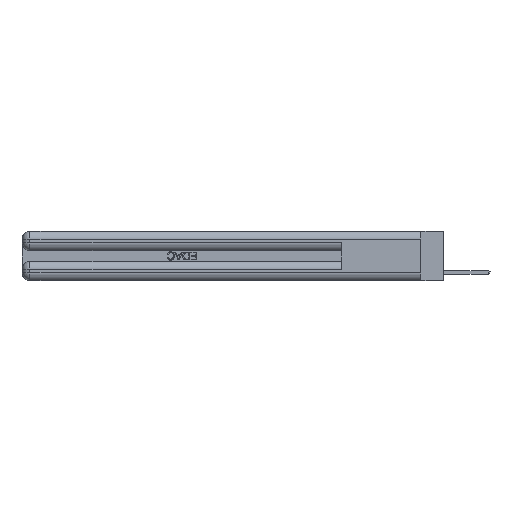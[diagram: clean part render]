
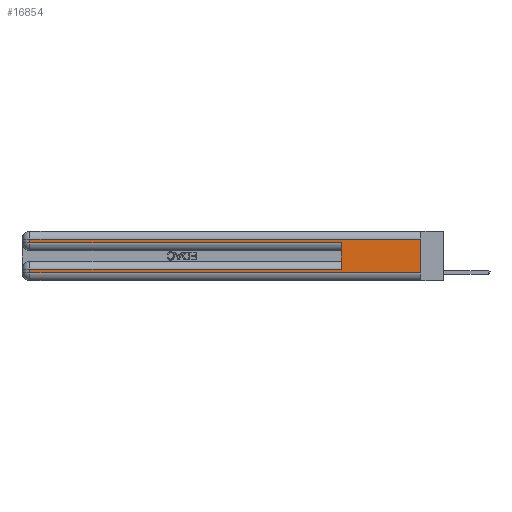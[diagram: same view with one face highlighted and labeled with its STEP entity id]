
A CAD part, left-side view. The second image highlights one B-rep face of the part: STEP entity #16854.
In plain terms, the highlighted planar face has unit normal (-1, 0, 0).
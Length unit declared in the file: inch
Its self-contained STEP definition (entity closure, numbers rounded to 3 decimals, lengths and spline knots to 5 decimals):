
#321 = VECTOR ( 'NONE', #23552, 39.37008 ) ;
#408 = DIRECTION ( 'NONE',  ( 0., 0., -1. ) ) ;
#588 = VERTEX_POINT ( 'NONE', #6368 ) ;
#1435 = DIRECTION ( 'NONE',  ( 0., 0., -1. ) ) ;
#3565 = CARTESIAN_POINT ( 'NONE',  ( 0., 2.94, 0.085 ) ) ;
#5109 = LINE ( 'NONE', #9982, #24723 ) ;
#5563 = EDGE_CURVE ( 'NONE', #7934, #24191, #11247, .T. ) ;
#6368 = CARTESIAN_POINT ( 'NONE',  ( 0., 2.94, 0.285 ) ) ;
#6643 = DIRECTION ( 'NONE',  ( 1., 0., 0. ) ) ;
#6859 = VECTOR ( 'NONE', #1435, 39.37008 ) ;
#7024 = LINE ( 'NONE', #15094, #10107 ) ;
#7531 = CARTESIAN_POINT ( 'NONE',  ( 0., 2.94, 0.37 ) ) ;
#7588 = LINE ( 'NONE', #26789, #12062 ) ;
#7934 = VERTEX_POINT ( 'NONE', #3565 ) ;
#8549 = EDGE_CURVE ( 'NONE', #28459, #16410, #17909, .T. ) ;
#9051 = PLANE ( 'NONE',  #22265 ) ;
#9515 = VECTOR ( 'NONE', #25153, 39.37008 ) ;
#9982 = CARTESIAN_POINT ( 'NONE',  ( 0., 0., 0.06 ) ) ;
#10107 = VECTOR ( 'NONE', #15269, 39.37008 ) ;
#10174 = CARTESIAN_POINT ( 'NONE',  ( 0., 0.6, 0.285 ) ) ;
#10999 = VECTOR ( 'NONE', #17253, 39.37008 ) ;
#11247 = LINE ( 'NONE', #24869, #9515 ) ;
#11629 = LINE ( 'NONE', #7531, #6859 ) ;
#12062 = VECTOR ( 'NONE', #18095, 39.37008 ) ;
#12458 = CARTESIAN_POINT ( 'NONE',  ( 0., 2.94, 0.31 ) ) ;
#13472 = CARTESIAN_POINT ( 'NONE',  ( 0., 0., 0.37 ) ) ;
#14002 = ORIENTED_EDGE ( 'NONE', *, *, #25707, .T. ) ;
#14356 = CARTESIAN_POINT ( 'NONE',  ( 0., 0., 0.06 ) ) ;
#15094 = CARTESIAN_POINT ( 'NONE',  ( 0., 0., 0.285 ) ) ;
#15269 = DIRECTION ( 'NONE',  ( 0., -1., 0. ) ) ;
#15651 = VERTEX_POINT ( 'NONE', #23390 ) ;
#15902 = ORIENTED_EDGE ( 'NONE', *, *, #28326, .T. ) ;
#16410 = VERTEX_POINT ( 'NONE', #10174 ) ;
#16618 = ORIENTED_EDGE ( 'NONE', *, *, #28120, .T. ) ;
#16854 = ADVANCED_FACE ( 'NONE', ( #20626 ), #9051, .F. ) ;
#17140 = EDGE_CURVE ( 'NONE', #24191, #18978, #5109, .T. ) ;
#17253 = DIRECTION ( 'NONE',  ( 0., 0., 1. ) ) ;
#17909 = LINE ( 'NONE', #21868, #10999 ) ;
#17926 = LINE ( 'NONE', #21050, #321 ) ;
#18095 = DIRECTION ( 'NONE',  ( 0., 1., 0. ) ) ;
#18299 = ORIENTED_EDGE ( 'NONE', *, *, #26901, .F. ) ;
#18856 = ORIENTED_EDGE ( 'NONE', *, *, #8549, .F. ) ;
#18978 = VERTEX_POINT ( 'NONE', #14356 ) ;
#19306 = LINE ( 'NONE', #22376, #26174 ) ;
#19713 = DIRECTION ( 'NONE',  ( 0., 0., -1. ) ) ;
#20626 = FACE_OUTER_BOUND ( 'NONE', #26253, .T. ) ;
#21050 = CARTESIAN_POINT ( 'NONE',  ( 0., 0., 0.085 ) ) ;
#21868 = CARTESIAN_POINT ( 'NONE',  ( 0., 0.6, 0.145 ) ) ;
#22265 = AXIS2_PLACEMENT_3D ( 'NONE', #13472, #6643, #19713 ) ;
#22360 = EDGE_CURVE ( 'NONE', #24361, #588, #11629, .T. ) ;
#22376 = CARTESIAN_POINT ( 'NONE',  ( 0., 0., 0.37 ) ) ;
#23390 = CARTESIAN_POINT ( 'NONE',  ( 0., 0., 0.31 ) ) ;
#23552 = DIRECTION ( 'NONE',  ( 0., 1., 0. ) ) ;
#24191 = VERTEX_POINT ( 'NONE', #26840 ) ;
#24361 = VERTEX_POINT ( 'NONE', #12458 ) ;
#24723 = VECTOR ( 'NONE', #27804, 39.37008 ) ;
#24814 = ORIENTED_EDGE ( 'NONE', *, *, #22360, .T. ) ;
#24869 = CARTESIAN_POINT ( 'NONE',  ( 0., 2.94, 0.37 ) ) ;
#25153 = DIRECTION ( 'NONE',  ( 0., 0., -1. ) ) ;
#25707 = EDGE_CURVE ( 'NONE', #588, #16410, #7024, .T. ) ;
#26115 = CARTESIAN_POINT ( 'NONE',  ( 0., 0.6, 0.085 ) ) ;
#26151 = ORIENTED_EDGE ( 'NONE', *, *, #5563, .T. ) ;
#26174 = VECTOR ( 'NONE', #408, 39.37008 ) ;
#26253 = EDGE_LOOP ( 'NONE', ( #18299, #16618, #24814, #14002, #18856, #15902, #26151, #26421 ) ) ;
#26421 = ORIENTED_EDGE ( 'NONE', *, *, #17140, .T. ) ;
#26789 = CARTESIAN_POINT ( 'NONE',  ( 0., 0., 0.31 ) ) ;
#26840 = CARTESIAN_POINT ( 'NONE',  ( 0., 2.94, 0.06 ) ) ;
#26901 = EDGE_CURVE ( 'NONE', #15651, #18978, #19306, .T. ) ;
#27804 = DIRECTION ( 'NONE',  ( 0., -1., 0. ) ) ;
#28120 = EDGE_CURVE ( 'NONE', #15651, #24361, #7588, .T. ) ;
#28326 = EDGE_CURVE ( 'NONE', #28459, #7934, #17926, .T. ) ;
#28459 = VERTEX_POINT ( 'NONE', #26115 ) ;
